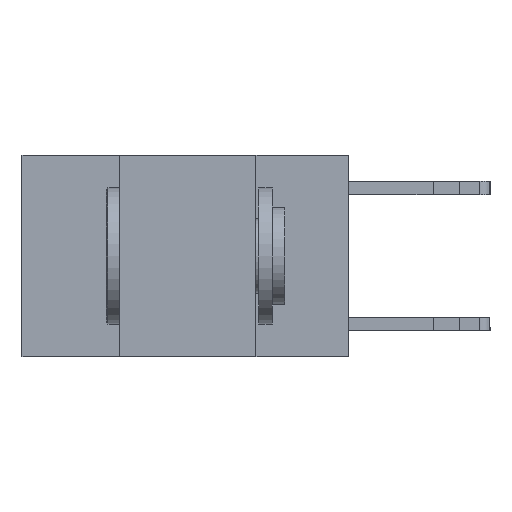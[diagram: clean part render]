
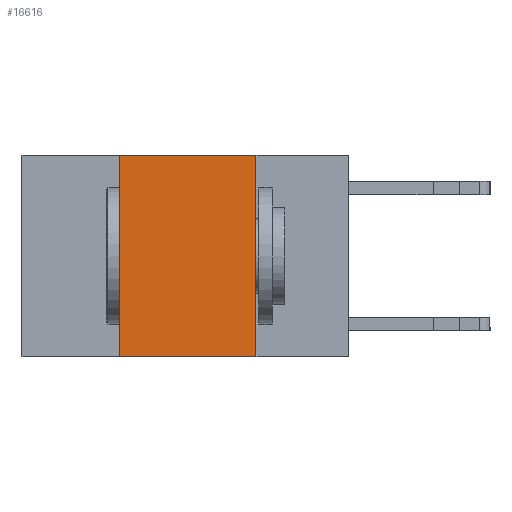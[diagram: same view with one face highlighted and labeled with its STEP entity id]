
A CAD part, left-side view. The second image highlights one B-rep face of the part: STEP entity #16616.
In plain terms, the highlighted planar face has unit normal (-1, 0, 0).
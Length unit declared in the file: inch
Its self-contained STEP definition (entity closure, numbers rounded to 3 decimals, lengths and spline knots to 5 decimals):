
#1678 = DIRECTION ( 'NONE',  ( 0., 0., -1. ) ) ;
#1856 = DIRECTION ( 'NONE',  ( 0., 0., -1. ) ) ;
#1992 = DIRECTION ( 'NONE',  ( 0., 0., 1. ) ) ;
#2213 = VECTOR ( 'NONE', #3342, 39.37008 ) ;
#3215 = EDGE_CURVE ( 'NONE', #7862, #11264, #4698, .T. ) ;
#3342 = DIRECTION ( 'NONE',  ( 0., -1., 0. ) ) ;
#3431 = VERTEX_POINT ( 'NONE', #7657 ) ;
#3523 = ORIENTED_EDGE ( 'NONE', *, *, #3215, .F. ) ;
#4321 = CARTESIAN_POINT ( 'NONE',  ( 0., 0.6, 0. ) ) ;
#4409 = FACE_OUTER_BOUND ( 'NONE', #5954, .T. ) ;
#4698 = LINE ( 'NONE', #5623, #2213 ) ;
#4836 = LINE ( 'NONE', #12743, #7796 ) ;
#5623 = CARTESIAN_POINT ( 'NONE',  ( 0., 0.6, 0. ) ) ;
#5954 = EDGE_LOOP ( 'NONE', ( #15630, #3523, #6065, #15657 ) ) ;
#6065 = ORIENTED_EDGE ( 'NONE', *, *, #12369, .F. ) ;
#6141 = CARTESIAN_POINT ( 'NONE',  ( 0., 0.42, 0. ) ) ;
#6279 = DIRECTION ( 'NONE',  ( 0., -1., 0. ) ) ;
#6396 = VECTOR ( 'NONE', #1992, 39.37008 ) ;
#7657 = CARTESIAN_POINT ( 'NONE',  ( 0., 0.42, -0.37 ) ) ;
#7667 = CARTESIAN_POINT ( 'NONE',  ( 0., 0.42, 0. ) ) ;
#7796 = VECTOR ( 'NONE', #6279, 39.37008 ) ;
#7808 = AXIS2_PLACEMENT_3D ( 'NONE', #4321, #9497, #1856 ) ;
#7862 = VERTEX_POINT ( 'NONE', #7667 ) ;
#9497 = DIRECTION ( 'NONE',  ( 1., 0., 0. ) ) ;
#10202 = EDGE_CURVE ( 'NONE', #11264, #15638, #10672, .T. ) ;
#10543 = CARTESIAN_POINT ( 'NONE',  ( 0., 0.17, 0. ) ) ;
#10672 = LINE ( 'NONE', #16008, #15218 ) ;
#10996 = CARTESIAN_POINT ( 'NONE',  ( 0., 0.17, -0.37 ) ) ;
#11264 = VERTEX_POINT ( 'NONE', #10543 ) ;
#12280 = LINE ( 'NONE', #6141, #6396 ) ;
#12369 = EDGE_CURVE ( 'NONE', #3431, #7862, #12280, .T. ) ;
#12743 = CARTESIAN_POINT ( 'NONE',  ( 0., 0.6, -0.37 ) ) ;
#14722 = EDGE_CURVE ( 'NONE', #3431, #15638, #4836, .T. ) ;
#15218 = VECTOR ( 'NONE', #1678, 39.37008 ) ;
#15630 = ORIENTED_EDGE ( 'NONE', *, *, #10202, .F. ) ;
#15638 = VERTEX_POINT ( 'NONE', #10996 ) ;
#15657 = ORIENTED_EDGE ( 'NONE', *, *, #14722, .T. ) ;
#15943 = PLANE ( 'NONE',  #7808 ) ;
#16008 = CARTESIAN_POINT ( 'NONE',  ( 0., 0.17, 0. ) ) ;
#16616 = ADVANCED_FACE ( 'NONE', ( #4409 ), #15943, .F. ) ;
